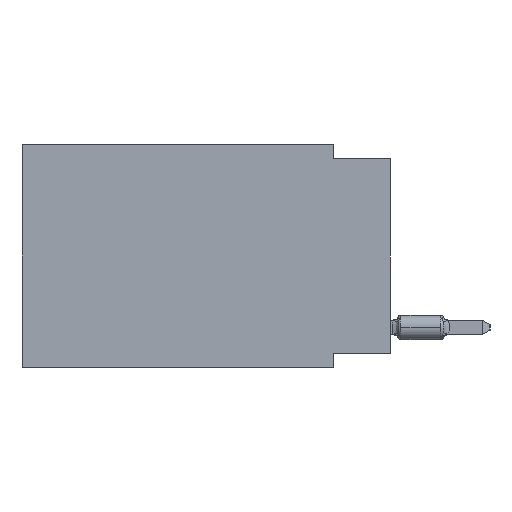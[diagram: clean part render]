
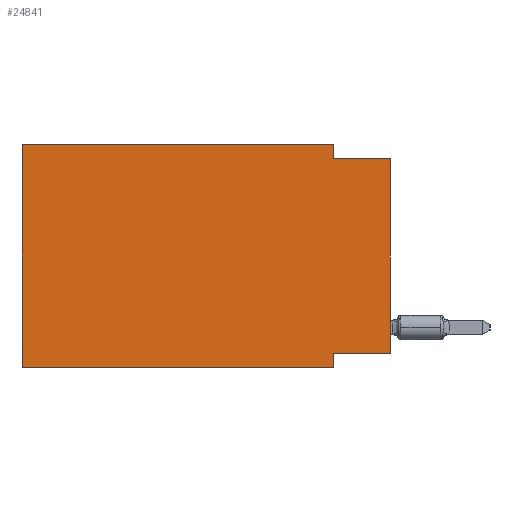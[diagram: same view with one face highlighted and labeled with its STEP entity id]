
A CAD part, left-side view. The second image highlights one B-rep face of the part: STEP entity #24841.
In plain terms, the highlighted planar face has unit normal (-1, 0, 0).
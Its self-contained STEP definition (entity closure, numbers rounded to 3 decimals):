
#631 = ORIENTED_EDGE ( 'NONE', *, *, #11909, .F. ) ;
#1146 = AXIS2_PLACEMENT_3D ( 'NONE', #12708, #1471, #16721 ) ;
#1471 = DIRECTION ( 'NONE',  ( 1., 0., 0. ) ) ;
#1611 = EDGE_CURVE ( 'NONE', #28080, #12315, #15143, .T. ) ;
#1796 = CARTESIAN_POINT ( 'NONE',  ( 0., 2.54, -9.271 ) ) ;
#2226 = VERTEX_POINT ( 'NONE', #27502 ) ;
#3529 = ORIENTED_EDGE ( 'NONE', *, *, #12594, .T. ) ;
#3604 = LINE ( 'NONE', #8179, #7763 ) ;
#3675 = LINE ( 'NONE', #12696, #4116 ) ;
#4116 = VECTOR ( 'NONE', #7971, 1000. ) ;
#4175 = LINE ( 'NONE', #6536, #18443 ) ;
#4219 = VERTEX_POINT ( 'NONE', #21625 ) ;
#5777 = CARTESIAN_POINT ( 'NONE',  ( 0., 0., -9.271 ) ) ;
#5956 = CARTESIAN_POINT ( 'NONE',  ( 0., 16.383, -9.906 ) ) ;
#6069 = EDGE_LOOP ( 'NONE', ( #25484, #16095, #8983, #631, #12208, #3529, #21229, #27528 ) ) ;
#6255 = LINE ( 'NONE', #19737, #17600 ) ;
#6536 = CARTESIAN_POINT ( 'NONE',  ( 0., 0., 0. ) ) ;
#6986 = CARTESIAN_POINT ( 'NONE',  ( 0., 0., -0.635 ) ) ;
#7750 = DIRECTION ( 'NONE',  ( 0., -1., 0. ) ) ;
#7763 = VECTOR ( 'NONE', #7750, 1000. ) ;
#7971 = DIRECTION ( 'NONE',  ( 0., 0., 1. ) ) ;
#8179 = CARTESIAN_POINT ( 'NONE',  ( 0., 16.383, -9.906 ) ) ;
#8721 = EDGE_CURVE ( 'NONE', #12624, #25709, #3675, .T. ) ;
#8983 = ORIENTED_EDGE ( 'NONE', *, *, #23605, .F. ) ;
#11909 = EDGE_CURVE ( 'NONE', #25709, #4219, #17722, .T. ) ;
#12208 = ORIENTED_EDGE ( 'NONE', *, *, #8721, .F. ) ;
#12274 = CARTESIAN_POINT ( 'NONE',  ( 0., 2.54, 0. ) ) ;
#12315 = VERTEX_POINT ( 'NONE', #29209 ) ;
#12594 = EDGE_CURVE ( 'NONE', #12624, #12315, #3604, .T. ) ;
#12624 = VERTEX_POINT ( 'NONE', #5956 ) ;
#12696 = CARTESIAN_POINT ( 'NONE',  ( 0., 16.383, 0. ) ) ;
#12708 = CARTESIAN_POINT ( 'NONE',  ( 0., 16.383, 0. ) ) ;
#13113 = DIRECTION ( 'NONE',  ( 0., 0., -1. ) ) ;
#14495 = LINE ( 'NONE', #12274, #26236 ) ;
#15143 = LINE ( 'NONE', #24175, #25410 ) ;
#16014 = DIRECTION ( 'NONE',  ( 0., -1., 0. ) ) ;
#16095 = ORIENTED_EDGE ( 'NONE', *, *, #23168, .F. ) ;
#16600 = LINE ( 'NONE', #6986, #24343 ) ;
#16721 = DIRECTION ( 'NONE',  ( 0., 0., -1. ) ) ;
#17506 = DIRECTION ( 'NONE',  ( 0., 1., 0. ) ) ;
#17600 = VECTOR ( 'NONE', #17506, 1000. ) ;
#17722 = LINE ( 'NONE', #28944, #25689 ) ;
#18443 = VECTOR ( 'NONE', #26513, 1000. ) ;
#19715 = CARTESIAN_POINT ( 'NONE',  ( 0., 16.383, 0. ) ) ;
#19737 = CARTESIAN_POINT ( 'NONE',  ( 0., 0., -9.271 ) ) ;
#20408 = EDGE_CURVE ( 'NONE', #26389, #27394, #4175, .T. ) ;
#21229 = ORIENTED_EDGE ( 'NONE', *, *, #1611, .F. ) ;
#21473 = FACE_OUTER_BOUND ( 'NONE', #6069, .T. ) ;
#21625 = CARTESIAN_POINT ( 'NONE',  ( 0., 2.54, 0. ) ) ;
#21966 = DIRECTION ( 'NONE',  ( 0., 0., -1. ) ) ;
#22108 = EDGE_CURVE ( 'NONE', #26389, #28080, #6255, .T. ) ;
#23010 = CARTESIAN_POINT ( 'NONE',  ( 0., 0., -0.635 ) ) ;
#23168 = EDGE_CURVE ( 'NONE', #2226, #27394, #16600, .T. ) ;
#23605 = EDGE_CURVE ( 'NONE', #4219, #2226, #14495, .T. ) ;
#24175 = CARTESIAN_POINT ( 'NONE',  ( 0., 2.54, -9.906 ) ) ;
#24343 = VECTOR ( 'NONE', #16014, 1000. ) ;
#24841 = ADVANCED_FACE ( 'NONE', ( #21473 ), #26317, .F. ) ;
#25410 = VECTOR ( 'NONE', #21966, 1000. ) ;
#25484 = ORIENTED_EDGE ( 'NONE', *, *, #20408, .T. ) ;
#25689 = VECTOR ( 'NONE', #26587, 1000. ) ;
#25709 = VERTEX_POINT ( 'NONE', #19715 ) ;
#26236 = VECTOR ( 'NONE', #13113, 1000. ) ;
#26317 = PLANE ( 'NONE',  #1146 ) ;
#26389 = VERTEX_POINT ( 'NONE', #5777 ) ;
#26513 = DIRECTION ( 'NONE',  ( 0., 0., 1. ) ) ;
#26587 = DIRECTION ( 'NONE',  ( 0., -1., 0. ) ) ;
#27394 = VERTEX_POINT ( 'NONE', #23010 ) ;
#27502 = CARTESIAN_POINT ( 'NONE',  ( 0., 2.54, -0.635 ) ) ;
#27528 = ORIENTED_EDGE ( 'NONE', *, *, #22108, .F. ) ;
#28080 = VERTEX_POINT ( 'NONE', #1796 ) ;
#28944 = CARTESIAN_POINT ( 'NONE',  ( 0., 16.383, 0. ) ) ;
#29209 = CARTESIAN_POINT ( 'NONE',  ( 0., 2.54, -9.906 ) ) ;
